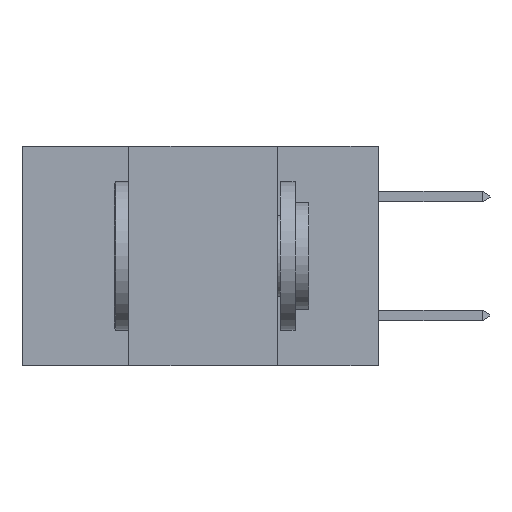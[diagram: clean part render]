
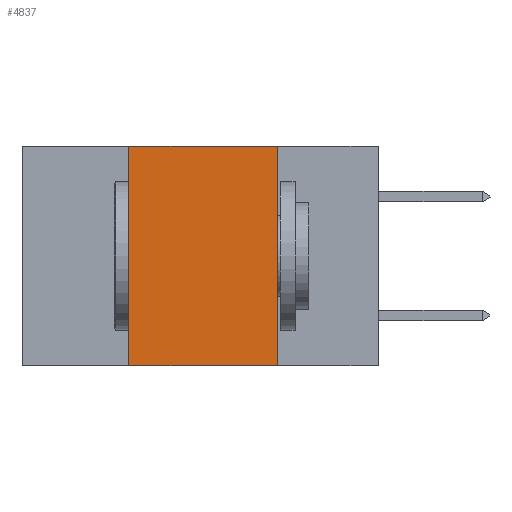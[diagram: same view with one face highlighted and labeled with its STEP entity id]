
A CAD part, left-side view. The second image highlights one B-rep face of the part: STEP entity #4837.
In plain terms, the highlighted planar face has unit normal (-1, 0, 0).
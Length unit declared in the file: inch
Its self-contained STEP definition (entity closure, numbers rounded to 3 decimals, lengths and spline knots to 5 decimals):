
#200 = ORIENTED_EDGE ( 'NONE', *, *, #14720, .F. ) ;
#3806 = PLANE ( 'NONE',  #21236 ) ;
#4837 = ADVANCED_FACE ( 'NONE', ( #19960 ), #3806, .F. ) ;
#8658 = DIRECTION ( 'NONE',  ( 0., 0., -1. ) ) ;
#8737 = DIRECTION ( 'NONE',  ( 0., 0., -1. ) ) ;
#9857 = EDGE_CURVE ( 'NONE', #30052, #13446, #24457, .T. ) ;
#9945 = VERTEX_POINT ( 'NONE', #16791 ) ;
#9998 = LINE ( 'NONE', #30588, #10746 ) ;
#10333 = VECTOR ( 'NONE', #27551, 39.37008 ) ;
#10746 = VECTOR ( 'NONE', #8658, 39.37008 ) ;
#11512 = CARTESIAN_POINT ( 'NONE',  ( 0., 0.42, 0. ) ) ;
#12289 = VECTOR ( 'NONE', #26261, 39.37008 ) ;
#13121 = DIRECTION ( 'NONE',  ( 0., -1., 0. ) ) ;
#13446 = VERTEX_POINT ( 'NONE', #11512 ) ;
#13805 = LINE ( 'NONE', #30169, #25962 ) ;
#14625 = EDGE_CURVE ( 'NONE', #13446, #9945, #13805, .T. ) ;
#14720 = EDGE_CURVE ( 'NONE', #9945, #21835, #9998, .T. ) ;
#16791 = CARTESIAN_POINT ( 'NONE',  ( 0., 0.17, 0. ) ) ;
#19960 = FACE_OUTER_BOUND ( 'NONE', #27722, .T. ) ;
#20794 = ORIENTED_EDGE ( 'NONE', *, *, #30637, .T. ) ;
#20852 = CARTESIAN_POINT ( 'NONE',  ( 0., 0.6, 0. ) ) ;
#21160 = ORIENTED_EDGE ( 'NONE', *, *, #14625, .F. ) ;
#21236 = AXIS2_PLACEMENT_3D ( 'NONE', #20852, #23311, #8737 ) ;
#21835 = VERTEX_POINT ( 'NONE', #25194 ) ;
#22646 = CARTESIAN_POINT ( 'NONE',  ( 0., 0.6, -0.37 ) ) ;
#23010 = CARTESIAN_POINT ( 'NONE',  ( 0., 0.42, -0.37 ) ) ;
#23267 = LINE ( 'NONE', #22646, #10333 ) ;
#23311 = DIRECTION ( 'NONE',  ( 1., 0., 0. ) ) ;
#23463 = ORIENTED_EDGE ( 'NONE', *, *, #9857, .F. ) ;
#24457 = LINE ( 'NONE', #31177, #12289 ) ;
#25194 = CARTESIAN_POINT ( 'NONE',  ( 0., 0.17, -0.37 ) ) ;
#25962 = VECTOR ( 'NONE', #13121, 39.37008 ) ;
#26261 = DIRECTION ( 'NONE',  ( 0., 0., 1. ) ) ;
#27551 = DIRECTION ( 'NONE',  ( 0., -1., 0. ) ) ;
#27722 = EDGE_LOOP ( 'NONE', ( #200, #21160, #23463, #20794 ) ) ;
#30052 = VERTEX_POINT ( 'NONE', #23010 ) ;
#30169 = CARTESIAN_POINT ( 'NONE',  ( 0., 0.6, 0. ) ) ;
#30588 = CARTESIAN_POINT ( 'NONE',  ( 0., 0.17, 0. ) ) ;
#30637 = EDGE_CURVE ( 'NONE', #30052, #21835, #23267, .T. ) ;
#31177 = CARTESIAN_POINT ( 'NONE',  ( 0., 0.42, 0. ) ) ;
